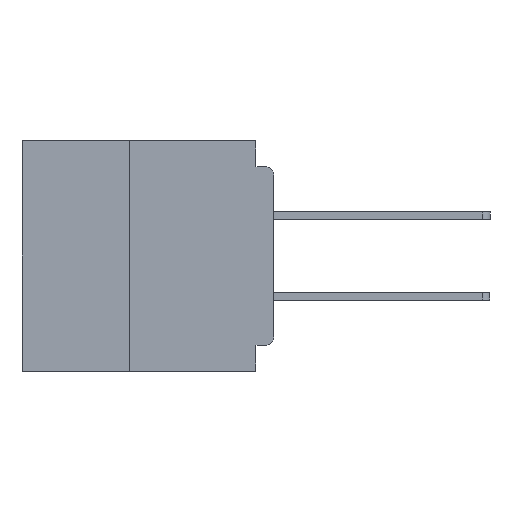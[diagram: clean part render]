
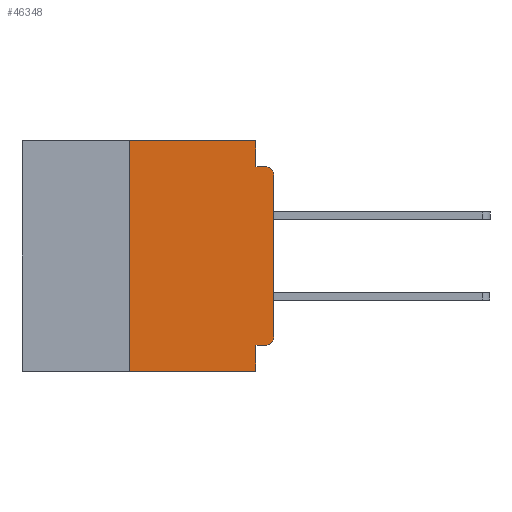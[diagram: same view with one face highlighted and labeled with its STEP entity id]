
A CAD part, left-side view. The second image highlights one B-rep face of the part: STEP entity #46348.
In plain terms, the highlighted planar face has unit normal (-1, 0, 0).
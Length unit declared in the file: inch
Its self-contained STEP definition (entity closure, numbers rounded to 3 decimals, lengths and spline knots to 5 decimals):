
#1070 = DIRECTION ( 'NONE',  ( 0., 0., -1. ) ) ;
#1480 = ORIENTED_EDGE ( 'NONE', *, *, #26067, .T. ) ;
#1683 = VERTEX_POINT ( 'NONE', #37046 ) ;
#2623 = CARTESIAN_POINT ( 'NONE',  ( 0., 0.031, 0. ) ) ;
#3245 = ORIENTED_EDGE ( 'NONE', *, *, #40511, .F. ) ;
#6060 = ORIENTED_EDGE ( 'NONE', *, *, #31510, .F. ) ;
#6768 = CARTESIAN_POINT ( 'NONE',  ( 0., 0., -0.34 ) ) ;
#7085 = EDGE_CURVE ( 'NONE', #17759, #32598, #41222, .T. ) ;
#7608 = CARTESIAN_POINT ( 'NONE',  ( 0., 0., -0.06 ) ) ;
#7962 = VERTEX_POINT ( 'NONE', #6768 ) ;
#7972 = VERTEX_POINT ( 'NONE', #35787 ) ;
#8087 = DIRECTION ( 'NONE',  ( 0., 0., -1. ) ) ;
#10512 = EDGE_CURVE ( 'NONE', #32939, #7972, #46517, .T. ) ;
#11063 = VERTEX_POINT ( 'NONE', #2623 ) ;
#11196 = ORIENTED_EDGE ( 'NONE', *, *, #10512, .F. ) ;
#11926 = CARTESIAN_POINT ( 'NONE',  ( 0., 0.031, 0. ) ) ;
#11995 = VECTOR ( 'NONE', #17748, 39.37008 ) ;
#12254 = DIRECTION ( 'NONE',  ( -1., 0., 0. ) ) ;
#12355 = CARTESIAN_POINT ( 'NONE',  ( 0., 0.031, -0.045 ) ) ;
#12916 = ORIENTED_EDGE ( 'NONE', *, *, #21215, .T. ) ;
#13580 = LINE ( 'NONE', #21996, #22178 ) ;
#14082 = CARTESIAN_POINT ( 'NONE',  ( 0., 0., 0. ) ) ;
#14251 = CARTESIAN_POINT ( 'NONE',  ( 0., 0.25, -0.4 ) ) ;
#14294 = LINE ( 'NONE', #14082, #11995 ) ;
#14303 = DIRECTION ( 'NONE',  ( 0., -1., 0. ) ) ;
#14643 = FACE_OUTER_BOUND ( 'NONE', #34681, .T. ) ;
#14878 = LINE ( 'NONE', #41258, #42599 ) ;
#16856 = EDGE_CURVE ( 'NONE', #32988, #32598, #19425, .T. ) ;
#17352 = CARTESIAN_POINT ( 'NONE',  ( 0., 0.031, -0.355 ) ) ;
#17435 = ORIENTED_EDGE ( 'NONE', *, *, #34836, .T. ) ;
#17748 = DIRECTION ( 'NONE',  ( 0., 0., 1. ) ) ;
#17759 = VERTEX_POINT ( 'NONE', #17352 ) ;
#18265 = VECTOR ( 'NONE', #43941, 39.37008 ) ;
#18318 = DIRECTION ( 'NONE',  ( 0., -1., 0. ) ) ;
#18447 = CIRCLE ( 'NONE', #23987, 0.015 ) ;
#18906 = VECTOR ( 'NONE', #14303, 39.37008 ) ;
#18985 = AXIS2_PLACEMENT_3D ( 'NONE', #34020, #12254, #37588 ) ;
#19221 = ORIENTED_EDGE ( 'NONE', *, *, #7085, .F. ) ;
#19425 = LINE ( 'NONE', #22408, #18265 ) ;
#19927 = AXIS2_PLACEMENT_3D ( 'NONE', #22590, #29887, #8087 ) ;
#20643 = CIRCLE ( 'NONE', #18985, 0.015 ) ;
#20644 = DIRECTION ( 'NONE',  ( -1., 0., 0. ) ) ;
#21215 = EDGE_CURVE ( 'NONE', #23038, #7962, #20643, .T. ) ;
#21746 = CARTESIAN_POINT ( 'NONE',  ( 0., 0.015, -0.355 ) ) ;
#21996 = CARTESIAN_POINT ( 'NONE',  ( 0., 0.437, 0. ) ) ;
#22178 = VECTOR ( 'NONE', #18318, 39.37008 ) ;
#22408 = CARTESIAN_POINT ( 'NONE',  ( 0., 0.437, -0.4 ) ) ;
#22590 = CARTESIAN_POINT ( 'NONE',  ( 0., 0.437, 0. ) ) ;
#22944 = CARTESIAN_POINT ( 'NONE',  ( 0., 0.031, -0.4 ) ) ;
#23038 = VERTEX_POINT ( 'NONE', #21746 ) ;
#23987 = AXIS2_PLACEMENT_3D ( 'NONE', #42218, #20644, #45848 ) ;
#26067 = EDGE_CURVE ( 'NONE', #36192, #7972, #18447, .T. ) ;
#26873 = CARTESIAN_POINT ( 'NONE',  ( 0., 0.25, -0.4 ) ) ;
#29887 = DIRECTION ( 'NONE',  ( 1., 0., 0. ) ) ;
#30545 = ORIENTED_EDGE ( 'NONE', *, *, #33872, .F. ) ;
#31510 = EDGE_CURVE ( 'NONE', #32988, #1683, #37827, .T. ) ;
#32598 = VERTEX_POINT ( 'NONE', #35542 ) ;
#32939 = VERTEX_POINT ( 'NONE', #12355 ) ;
#32988 = VERTEX_POINT ( 'NONE', #26873 ) ;
#33872 = EDGE_CURVE ( 'NONE', #11063, #32939, #35910, .T. ) ;
#34020 = CARTESIAN_POINT ( 'NONE',  ( 0., 0.015, -0.34 ) ) ;
#34681 = EDGE_LOOP ( 'NONE', ( #17435, #1480, #11196, #30545, #43437, #6060, #37253, #19221, #3245, #12916 ) ) ;
#34836 = EDGE_CURVE ( 'NONE', #7962, #36192, #14294, .T. ) ;
#35542 = CARTESIAN_POINT ( 'NONE',  ( 0., 0.031, -0.4 ) ) ;
#35787 = CARTESIAN_POINT ( 'NONE',  ( 0., 0.015, -0.045 ) ) ;
#35910 = LINE ( 'NONE', #11926, #45491 ) ;
#35931 = DIRECTION ( 'NONE',  ( 0., 0., 1. ) ) ;
#35986 = CARTESIAN_POINT ( 'NONE',  ( 0., 0., -0.045 ) ) ;
#36192 = VERTEX_POINT ( 'NONE', #7608 ) ;
#36914 = PLANE ( 'NONE',  #19927 ) ;
#37046 = CARTESIAN_POINT ( 'NONE',  ( 0., 0.25, 0. ) ) ;
#37238 = DIRECTION ( 'NONE',  ( 0., 0., -1. ) ) ;
#37253 = ORIENTED_EDGE ( 'NONE', *, *, #16856, .T. ) ;
#37588 = DIRECTION ( 'NONE',  ( 0., 0., -1. ) ) ;
#37827 = LINE ( 'NONE', #14251, #46263 ) ;
#40511 = EDGE_CURVE ( 'NONE', #23038, #17759, #14878, .T. ) ;
#41222 = LINE ( 'NONE', #22944, #42356 ) ;
#41258 = CARTESIAN_POINT ( 'NONE',  ( 0., 0., -0.355 ) ) ;
#42218 = CARTESIAN_POINT ( 'NONE',  ( 0., 0.015, -0.06 ) ) ;
#42356 = VECTOR ( 'NONE', #1070, 39.37008 ) ;
#42599 = VECTOR ( 'NONE', #44890, 39.37008 ) ;
#43437 = ORIENTED_EDGE ( 'NONE', *, *, #44793, .F. ) ;
#43941 = DIRECTION ( 'NONE',  ( 0., -1., 0. ) ) ;
#44793 = EDGE_CURVE ( 'NONE', #1683, #11063, #13580, .T. ) ;
#44890 = DIRECTION ( 'NONE',  ( 0., 1., 0. ) ) ;
#45491 = VECTOR ( 'NONE', #37238, 39.37008 ) ;
#45848 = DIRECTION ( 'NONE',  ( 0., 0., -1. ) ) ;
#46263 = VECTOR ( 'NONE', #35931, 39.37008 ) ;
#46348 = ADVANCED_FACE ( 'NONE', ( #14643 ), #36914, .F. ) ;
#46517 = LINE ( 'NONE', #35986, #18906 ) ;
